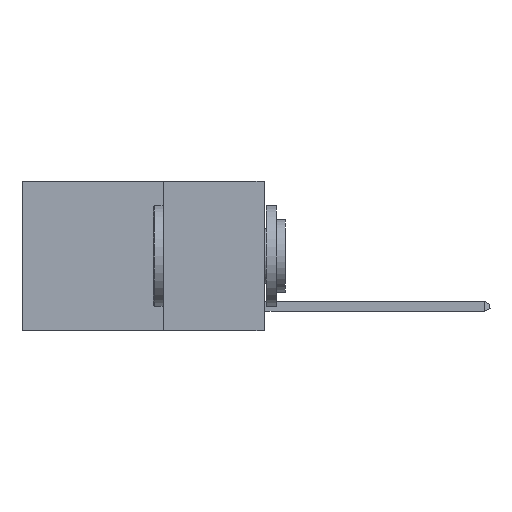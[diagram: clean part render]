
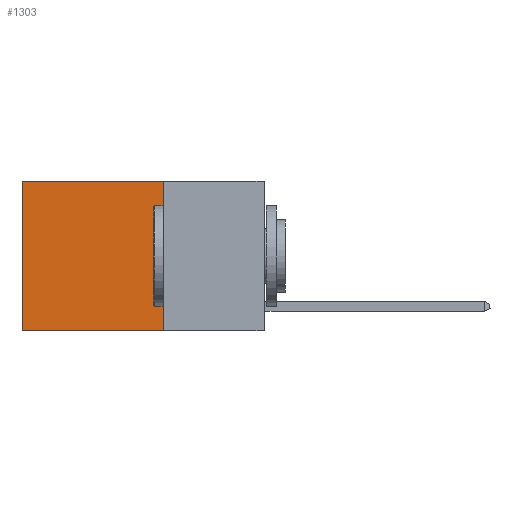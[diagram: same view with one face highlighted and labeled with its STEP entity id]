
A CAD part, left-side view. The second image highlights one B-rep face of the part: STEP entity #1303.
In plain terms, the highlighted planar face has unit normal (-1, 0, 0).
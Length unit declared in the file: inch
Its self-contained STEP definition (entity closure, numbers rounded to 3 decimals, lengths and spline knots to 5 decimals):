
#541 = CARTESIAN_POINT ( 'NONE',  ( 0.2625, 0.6, 0. ) ) ;
#1254 = CARTESIAN_POINT ( 'NONE',  ( 0.2625, 0.25, 0. ) ) ;
#1303 = ADVANCED_FACE ( 'NONE', ( #14784 ), #11328, .F. ) ;
#2164 = LINE ( 'NONE', #9003, #13329 ) ;
#2892 = DIRECTION ( 'NONE',  ( 1., 0., 0. ) ) ;
#3317 = CARTESIAN_POINT ( 'NONE',  ( 0.2625, 0.25, 0. ) ) ;
#3776 = CARTESIAN_POINT ( 'NONE',  ( 0.2625, 0.25, 0. ) ) ;
#4305 = CARTESIAN_POINT ( 'NONE',  ( 0.2625, 0.25, 0. ) ) ;
#4775 = VECTOR ( 'NONE', #4843, 39.37008 ) ;
#4843 = DIRECTION ( 'NONE',  ( 0., 1., 0. ) ) ;
#5747 = DIRECTION ( 'NONE',  ( 0., 0., -1. ) ) ;
#6002 = EDGE_CURVE ( 'NONE', #17673, #9447, #16731, .T. ) ;
#6230 = CARTESIAN_POINT ( 'NONE',  ( 0.2625, 0.25, -0.37 ) ) ;
#6938 = ORIENTED_EDGE ( 'NONE', *, *, #18224, .T. ) ;
#8731 = AXIS2_PLACEMENT_3D ( 'NONE', #4305, #2892, #9961 ) ;
#9003 = CARTESIAN_POINT ( 'NONE',  ( 0.2625, 0.6, 0. ) ) ;
#9237 = DIRECTION ( 'NONE',  ( 0., 0., -1. ) ) ;
#9351 = ORIENTED_EDGE ( 'NONE', *, *, #6002, .F. ) ;
#9447 = VERTEX_POINT ( 'NONE', #16047 ) ;
#9961 = DIRECTION ( 'NONE',  ( 0., 0., -1. ) ) ;
#11328 = PLANE ( 'NONE',  #8731 ) ;
#11414 = DIRECTION ( 'NONE',  ( 0., 1., 0. ) ) ;
#13153 = VERTEX_POINT ( 'NONE', #541 ) ;
#13329 = VECTOR ( 'NONE', #9237, 39.37008 ) ;
#14157 = LINE ( 'NONE', #3776, #17023 ) ;
#14784 = FACE_OUTER_BOUND ( 'NONE', #17104, .T. ) ;
#16047 = CARTESIAN_POINT ( 'NONE',  ( 0.2625, 0.6, -0.37 ) ) ;
#16501 = ORIENTED_EDGE ( 'NONE', *, *, #22029, .T. ) ;
#16731 = LINE ( 'NONE', #6230, #18968 ) ;
#16874 = CARTESIAN_POINT ( 'NONE',  ( 0.2625, 0.25, -0.37 ) ) ;
#17023 = VECTOR ( 'NONE', #5747, 39.37008 ) ;
#17104 = EDGE_LOOP ( 'NONE', ( #16501, #9351, #21267, #6938 ) ) ;
#17162 = EDGE_CURVE ( 'NONE', #18226, #17673, #14157, .T. ) ;
#17673 = VERTEX_POINT ( 'NONE', #16874 ) ;
#18224 = EDGE_CURVE ( 'NONE', #18226, #13153, #20075, .T. ) ;
#18226 = VERTEX_POINT ( 'NONE', #3317 ) ;
#18968 = VECTOR ( 'NONE', #11414, 39.37008 ) ;
#20075 = LINE ( 'NONE', #1254, #4775 ) ;
#21267 = ORIENTED_EDGE ( 'NONE', *, *, #17162, .F. ) ;
#22029 = EDGE_CURVE ( 'NONE', #13153, #9447, #2164, .T. ) ;
